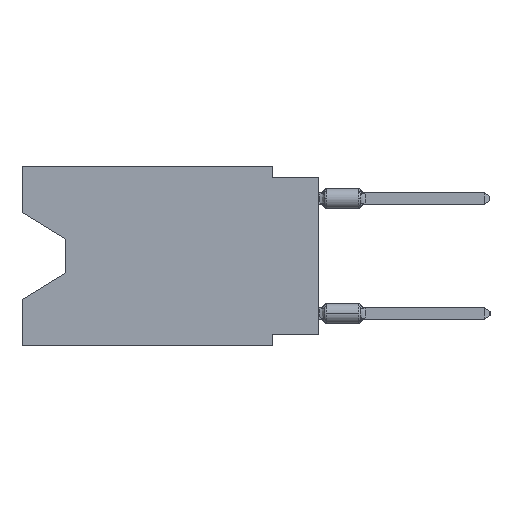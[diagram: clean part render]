
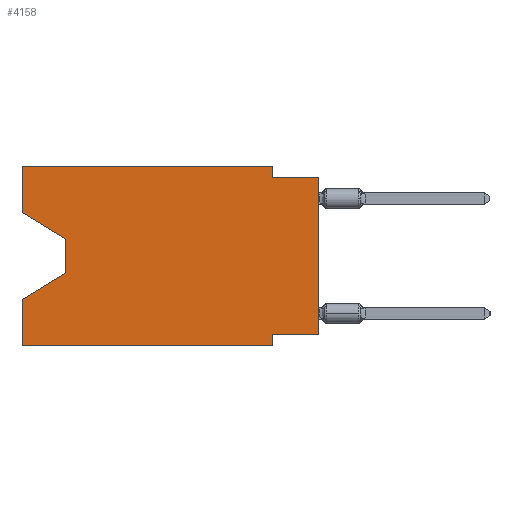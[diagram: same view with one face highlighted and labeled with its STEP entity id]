
A CAD part, left-side view. The second image highlights one B-rep face of the part: STEP entity #4158.
In plain terms, the highlighted planar face has unit normal (-1, 0, 0).
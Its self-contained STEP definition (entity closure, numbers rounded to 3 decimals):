
#132 = AXIS2_PLACEMENT_3D ( 'NONE', #12603, #7253, #28606 ) ;
#166 = EDGE_CURVE ( 'NONE', #31573, #31704, #13141, .T. ) ;
#570 = CARTESIAN_POINT ( 'NONE',  ( 0., 16.383, -7.36 ) ) ;
#793 = CARTESIAN_POINT ( 'NONE',  ( 0., 0., -0.635 ) ) ;
#852 = ORIENTED_EDGE ( 'NONE', *, *, #166, .F. ) ;
#869 = CARTESIAN_POINT ( 'NONE',  ( 0., 2.54, 0. ) ) ;
#1158 = DIRECTION ( 'NONE',  ( 0., 0., -1. ) ) ;
#1544 = CARTESIAN_POINT ( 'NONE',  ( 0., 0., -0.635 ) ) ;
#1701 = CARTESIAN_POINT ( 'NONE',  ( 0., 16.383, 0. ) ) ;
#1983 = VECTOR ( 'NONE', #14369, 1000. ) ;
#2043 = CARTESIAN_POINT ( 'NONE',  ( 0., 16.383, 0. ) ) ;
#2828 = LINE ( 'NONE', #10252, #24861 ) ;
#3545 = LINE ( 'NONE', #24716, #1983 ) ;
#3918 = CARTESIAN_POINT ( 'NONE',  ( 0., 13.97, -4.013 ) ) ;
#4142 = ORIENTED_EDGE ( 'NONE', *, *, #22416, .T. ) ;
#4158 = ADVANCED_FACE ( 'NONE', ( #22917 ), #33400, .F. ) ;
#5882 = ORIENTED_EDGE ( 'NONE', *, *, #30112, .F. ) ;
#6161 = ORIENTED_EDGE ( 'NONE', *, *, #25434, .T. ) ;
#6265 = CARTESIAN_POINT ( 'NONE',  ( 0., 13.97, -4.013 ) ) ;
#6303 = EDGE_CURVE ( 'NONE', #29428, #16116, #11948, .T. ) ;
#6849 = VERTEX_POINT ( 'NONE', #7433 ) ;
#6904 = VERTEX_POINT ( 'NONE', #869 ) ;
#7019 = VECTOR ( 'NONE', #17779, 1000. ) ;
#7045 = ORIENTED_EDGE ( 'NONE', *, *, #6303, .T. ) ;
#7253 = DIRECTION ( 'NONE',  ( 1., 0., 0. ) ) ;
#7433 = CARTESIAN_POINT ( 'NONE',  ( 0., 13.97, -5.893 ) ) ;
#7551 = LINE ( 'NONE', #2043, #10265 ) ;
#7754 = CARTESIAN_POINT ( 'NONE',  ( 0., 16.383, -9.906 ) ) ;
#8065 = VECTOR ( 'NONE', #11549, 1000. ) ;
#8219 = ORIENTED_EDGE ( 'NONE', *, *, #19337, .T. ) ;
#8267 = ORIENTED_EDGE ( 'NONE', *, *, #10152, .F. ) ;
#8386 = LINE ( 'NONE', #29381, #27849 ) ;
#9244 = VERTEX_POINT ( 'NONE', #570 ) ;
#9673 = CARTESIAN_POINT ( 'NONE',  ( 0., 0., -9.271 ) ) ;
#9677 = EDGE_CURVE ( 'NONE', #15655, #23866, #25286, .T. ) ;
#9965 = EDGE_CURVE ( 'NONE', #29428, #31796, #7551, .T. ) ;
#10152 = EDGE_CURVE ( 'NONE', #6904, #15655, #8386, .T. ) ;
#10252 = CARTESIAN_POINT ( 'NONE',  ( 0., 16.383, 0. ) ) ;
#10265 = VECTOR ( 'NONE', #17528, 1000. ) ;
#11302 = LINE ( 'NONE', #7754, #20856 ) ;
#11420 = VECTOR ( 'NONE', #14501, 1000. ) ;
#11549 = DIRECTION ( 'NONE',  ( 0., -1., 0. ) ) ;
#11948 = LINE ( 'NONE', #28292, #17857 ) ;
#12242 = VECTOR ( 'NONE', #29409, 1000. ) ;
#12603 = CARTESIAN_POINT ( 'NONE',  ( 0., 16.383, 0. ) ) ;
#13141 = LINE ( 'NONE', #20365, #7019 ) ;
#13592 = LINE ( 'NONE', #26663, #16718 ) ;
#13924 = CARTESIAN_POINT ( 'NONE',  ( 0., 2.54, -9.906 ) ) ;
#14369 = DIRECTION ( 'NONE',  ( 0., 0., 1. ) ) ;
#14501 = DIRECTION ( 'NONE',  ( 0., 0., -1. ) ) ;
#14742 = ORIENTED_EDGE ( 'NONE', *, *, #31678, .T. ) ;
#15655 = VERTEX_POINT ( 'NONE', #24190 ) ;
#15659 = CARTESIAN_POINT ( 'NONE',  ( 0., 2.54, -9.271 ) ) ;
#16116 = VERTEX_POINT ( 'NONE', #3918 ) ;
#16336 = ORIENTED_EDGE ( 'NONE', *, *, #16513, .F. ) ;
#16513 = EDGE_CURVE ( 'NONE', #32109, #9244, #3545, .T. ) ;
#16718 = VECTOR ( 'NONE', #31974, 1000. ) ;
#17004 = VECTOR ( 'NONE', #27201, 1000. ) ;
#17528 = DIRECTION ( 'NONE',  ( 0., 0., 1. ) ) ;
#17779 = DIRECTION ( 'NONE',  ( 0., 0., -1. ) ) ;
#17857 = VECTOR ( 'NONE', #24848, 1000. ) ;
#18985 = EDGE_CURVE ( 'NONE', #31796, #6904, #2828, .T. ) ;
#19337 = EDGE_CURVE ( 'NONE', #6849, #9244, #33422, .T. ) ;
#19778 = ORIENTED_EDGE ( 'NONE', *, *, #18985, .F. ) ;
#19957 = VERTEX_POINT ( 'NONE', #9673 ) ;
#20365 = CARTESIAN_POINT ( 'NONE',  ( 0., 2.54, -9.906 ) ) ;
#20856 = VECTOR ( 'NONE', #32094, 1000. ) ;
#21868 = EDGE_LOOP ( 'NONE', ( #7045, #6161, #8219, #16336, #4142, #852, #5882, #14742, #26239, #8267, #19778, #31224 ) ) ;
#22416 = EDGE_CURVE ( 'NONE', #32109, #31704, #11302, .T. ) ;
#22917 = FACE_OUTER_BOUND ( 'NONE', #21868, .T. ) ;
#23866 = VERTEX_POINT ( 'NONE', #793 ) ;
#24190 = CARTESIAN_POINT ( 'NONE',  ( 0., 2.54, -0.635 ) ) ;
#24215 = CARTESIAN_POINT ( 'NONE',  ( 0., 16.383, -9.906 ) ) ;
#24716 = CARTESIAN_POINT ( 'NONE',  ( 0., 16.383, 0. ) ) ;
#24848 = DIRECTION ( 'NONE',  ( 0., -0.855, -0.519 ) ) ;
#24861 = VECTOR ( 'NONE', #31390, 1000. ) ;
#25286 = LINE ( 'NONE', #1544, #8065 ) ;
#25434 = EDGE_CURVE ( 'NONE', #16116, #6849, #27251, .T. ) ;
#25900 = CARTESIAN_POINT ( 'NONE',  ( 0., 16.383, -2.546 ) ) ;
#26239 = ORIENTED_EDGE ( 'NONE', *, *, #9677, .F. ) ;
#26663 = CARTESIAN_POINT ( 'NONE',  ( 0., 0., 0. ) ) ;
#27201 = DIRECTION ( 'NONE',  ( 0., 1., 0. ) ) ;
#27251 = LINE ( 'NONE', #6265, #11420 ) ;
#27376 = CARTESIAN_POINT ( 'NONE',  ( 0., 0., -9.271 ) ) ;
#27849 = VECTOR ( 'NONE', #1158, 1000. ) ;
#28292 = CARTESIAN_POINT ( 'NONE',  ( 0., 16.383, -2.546 ) ) ;
#28606 = DIRECTION ( 'NONE',  ( 0., 0., -1. ) ) ;
#29381 = CARTESIAN_POINT ( 'NONE',  ( 0., 2.54, 0. ) ) ;
#29409 = DIRECTION ( 'NONE',  ( 0., 0.855, -0.519 ) ) ;
#29428 = VERTEX_POINT ( 'NONE', #25900 ) ;
#30112 = EDGE_CURVE ( 'NONE', #19957, #31573, #33023, .T. ) ;
#31224 = ORIENTED_EDGE ( 'NONE', *, *, #9965, .F. ) ;
#31390 = DIRECTION ( 'NONE',  ( 0., -1., 0. ) ) ;
#31573 = VERTEX_POINT ( 'NONE', #15659 ) ;
#31631 = CARTESIAN_POINT ( 'NONE',  ( 0., 13.97, -5.893 ) ) ;
#31678 = EDGE_CURVE ( 'NONE', #19957, #23866, #13592, .T. ) ;
#31704 = VERTEX_POINT ( 'NONE', #13924 ) ;
#31796 = VERTEX_POINT ( 'NONE', #1701 ) ;
#31974 = DIRECTION ( 'NONE',  ( 0., 0., 1. ) ) ;
#32094 = DIRECTION ( 'NONE',  ( 0., -1., 0. ) ) ;
#32109 = VERTEX_POINT ( 'NONE', #24215 ) ;
#33023 = LINE ( 'NONE', #27376, #17004 ) ;
#33400 = PLANE ( 'NONE',  #132 ) ;
#33422 = LINE ( 'NONE', #31631, #12242 ) ;
